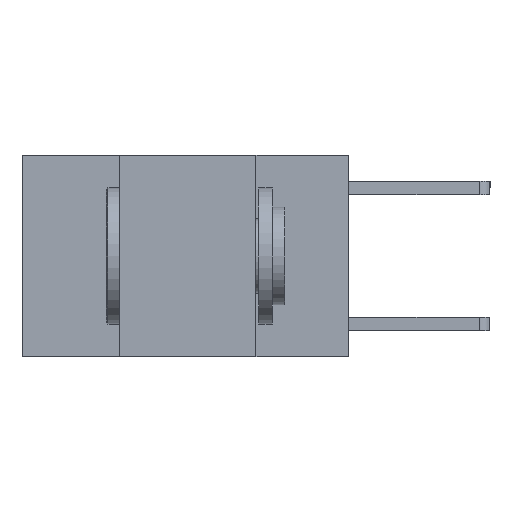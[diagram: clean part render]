
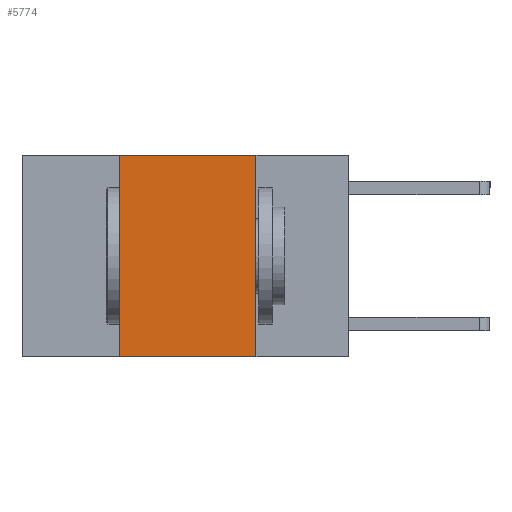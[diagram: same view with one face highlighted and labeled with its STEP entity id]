
A CAD part, left-side view. The second image highlights one B-rep face of the part: STEP entity #5774.
In plain terms, the highlighted planar face has unit normal (-1, 0, 0).
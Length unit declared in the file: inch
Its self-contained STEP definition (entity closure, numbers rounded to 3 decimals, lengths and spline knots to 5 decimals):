
#66 = VERTEX_POINT ( 'NONE', #4163 ) ;
#164 = DIRECTION ( 'NONE',  ( 0., 0., -1. ) ) ;
#178 = EDGE_CURVE ( 'NONE', #66, #4572, #8059, .T. ) ;
#283 = ORIENTED_EDGE ( 'NONE', *, *, #178, .F. ) ;
#546 = CARTESIAN_POINT ( 'NONE',  ( 0., 0.17, 0. ) ) ;
#604 = PLANE ( 'NONE',  #3049 ) ;
#881 = EDGE_CURVE ( 'NONE', #4572, #3293, #2287, .T. ) ;
#1417 = DIRECTION ( 'NONE',  ( 0., -1., 0. ) ) ;
#1966 = DIRECTION ( 'NONE',  ( 0., 0., 1. ) ) ;
#2076 = VERTEX_POINT ( 'NONE', #3985 ) ;
#2137 = CARTESIAN_POINT ( 'NONE',  ( 0., 0.17, 0. ) ) ;
#2287 = LINE ( 'NONE', #546, #8967 ) ;
#2852 = LINE ( 'NONE', #9289, #9484 ) ;
#2922 = CARTESIAN_POINT ( 'NONE',  ( 0., 0.17, -0.37 ) ) ;
#3049 = AXIS2_PLACEMENT_3D ( 'NONE', #9517, #7179, #164 ) ;
#3293 = VERTEX_POINT ( 'NONE', #2922 ) ;
#3457 = VECTOR ( 'NONE', #4628, 39.37008 ) ;
#3985 = CARTESIAN_POINT ( 'NONE',  ( 0., 0.42, -0.37 ) ) ;
#4163 = CARTESIAN_POINT ( 'NONE',  ( 0., 0.42, 0. ) ) ;
#4572 = VERTEX_POINT ( 'NONE', #2137 ) ;
#4628 = DIRECTION ( 'NONE',  ( 0., -1., 0. ) ) ;
#4792 = ORIENTED_EDGE ( 'NONE', *, *, #881, .F. ) ;
#5181 = EDGE_CURVE ( 'NONE', #2076, #3293, #6279, .T. ) ;
#5276 = VECTOR ( 'NONE', #1417, 39.37008 ) ;
#5377 = FACE_OUTER_BOUND ( 'NONE', #10385, .T. ) ;
#5774 = ADVANCED_FACE ( 'NONE', ( #5377 ), #604, .F. ) ;
#6279 = LINE ( 'NONE', #7732, #5276 ) ;
#6495 = ORIENTED_EDGE ( 'NONE', *, *, #9209, .F. ) ;
#6989 = ORIENTED_EDGE ( 'NONE', *, *, #5181, .T. ) ;
#7179 = DIRECTION ( 'NONE',  ( 1., 0., 0. ) ) ;
#7252 = CARTESIAN_POINT ( 'NONE',  ( 0., 0.6, 0. ) ) ;
#7732 = CARTESIAN_POINT ( 'NONE',  ( 0., 0.6, -0.37 ) ) ;
#8059 = LINE ( 'NONE', #7252, #3457 ) ;
#8870 = DIRECTION ( 'NONE',  ( 0., 0., -1. ) ) ;
#8967 = VECTOR ( 'NONE', #8870, 39.37008 ) ;
#9209 = EDGE_CURVE ( 'NONE', #2076, #66, #2852, .T. ) ;
#9289 = CARTESIAN_POINT ( 'NONE',  ( 0., 0.42, 0. ) ) ;
#9484 = VECTOR ( 'NONE', #1966, 39.37008 ) ;
#9517 = CARTESIAN_POINT ( 'NONE',  ( 0., 0.6, 0. ) ) ;
#10385 = EDGE_LOOP ( 'NONE', ( #4792, #283, #6495, #6989 ) ) ;
